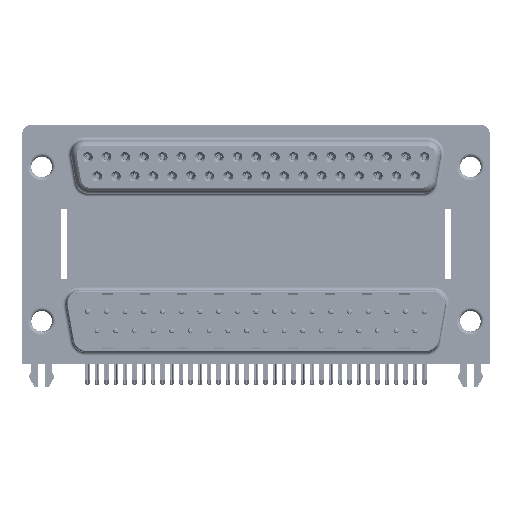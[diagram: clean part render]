
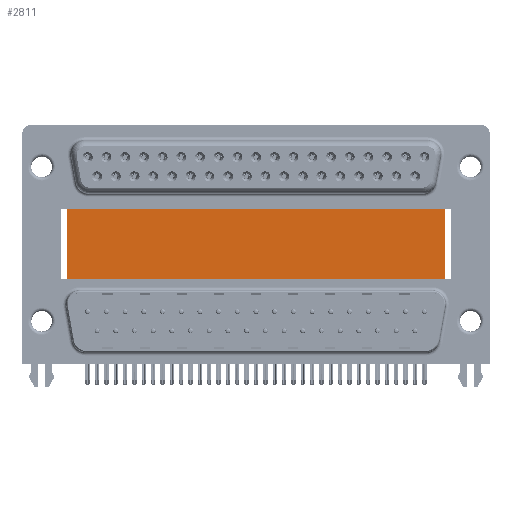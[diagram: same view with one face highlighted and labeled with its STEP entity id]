
A CAD part, top view. The second image highlights one B-rep face of the part: STEP entity #2811.
In plain terms, the highlighted planar face has unit normal (0, 0, 1).
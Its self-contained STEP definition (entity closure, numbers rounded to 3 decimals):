
#1091 = DIRECTION ( 'NONE',  ( 1., 0., 0. ) ) ;
#1386 = VECTOR ( 'NONE', #55073, 1000. ) ;
#1422 = DIRECTION ( 'NONE',  ( 0., 0., -1. ) ) ;
#1853 = DIRECTION ( 'NONE',  ( 1., 0., 0. ) ) ;
#2687 = CARTESIAN_POINT ( 'NONE',  ( 59.71, -3.735, -12. ) ) ;
#2811 = ADVANCED_FACE ( 'NONE', ( #47003 ), #51754, .F. ) ;
#2958 = EDGE_CURVE ( 'NONE', #9483, #5639, #26936, .T. ) ;
#5551 = CARTESIAN_POINT ( 'NONE',  ( 59.71, 16.585, -12. ) ) ;
#5639 = VERTEX_POINT ( 'NONE', #5551 ) ;
#7458 = EDGE_CURVE ( 'NONE', #9483, #9972, #65903, .T. ) ;
#9483 = VERTEX_POINT ( 'NONE', #59256 ) ;
#9972 = VERTEX_POINT ( 'NONE', #38497 ) ;
#12091 = LINE ( 'NONE', #43675, #19288 ) ;
#13629 = CARTESIAN_POINT ( 'NONE',  ( 3.79, 16.585, -12. ) ) ;
#15742 = CARTESIAN_POINT ( 'NONE',  ( 3.79, 16.585, -12. ) ) ;
#19288 = VECTOR ( 'NONE', #1853, 1000. ) ;
#20332 = VERTEX_POINT ( 'NONE', #2687 ) ;
#21325 = EDGE_LOOP ( 'NONE', ( #36403, #26288, #37103, #48367 ) ) ;
#24520 = VECTOR ( 'NONE', #1091, 1000. ) ;
#26288 = ORIENTED_EDGE ( 'NONE', *, *, #39059, .F. ) ;
#26936 = LINE ( 'NONE', #47676, #24520 ) ;
#32569 = AXIS2_PLACEMENT_3D ( 'NONE', #15742, #1422, #62260 ) ;
#36403 = ORIENTED_EDGE ( 'NONE', *, *, #54785, .T. ) ;
#37103 = ORIENTED_EDGE ( 'NONE', *, *, #2958, .F. ) ;
#38140 = CARTESIAN_POINT ( 'NONE',  ( 59.71, 16.585, -12. ) ) ;
#38497 = CARTESIAN_POINT ( 'NONE',  ( 3.79, -3.735, -12. ) ) ;
#39059 = EDGE_CURVE ( 'NONE', #5639, #20332, #65578, .T. ) ;
#43675 = CARTESIAN_POINT ( 'NONE',  ( 3.79, -3.735, -12. ) ) ;
#47003 = FACE_OUTER_BOUND ( 'NONE', #21325, .T. ) ;
#47055 = VECTOR ( 'NONE', #55081, 1000. ) ;
#47676 = CARTESIAN_POINT ( 'NONE',  ( 3.79, 16.585, -12. ) ) ;
#48367 = ORIENTED_EDGE ( 'NONE', *, *, #7458, .T. ) ;
#51754 = PLANE ( 'NONE',  #32569 ) ;
#54785 = EDGE_CURVE ( 'NONE', #9972, #20332, #12091, .T. ) ;
#55073 = DIRECTION ( 'NONE',  ( 0., -1., 0. ) ) ;
#55081 = DIRECTION ( 'NONE',  ( 0., -1., 0. ) ) ;
#59256 = CARTESIAN_POINT ( 'NONE',  ( 3.79, 16.585, -12. ) ) ;
#62260 = DIRECTION ( 'NONE',  ( -1., 0., 0. ) ) ;
#65578 = LINE ( 'NONE', #38140, #47055 ) ;
#65903 = LINE ( 'NONE', #13629, #1386 ) ;
